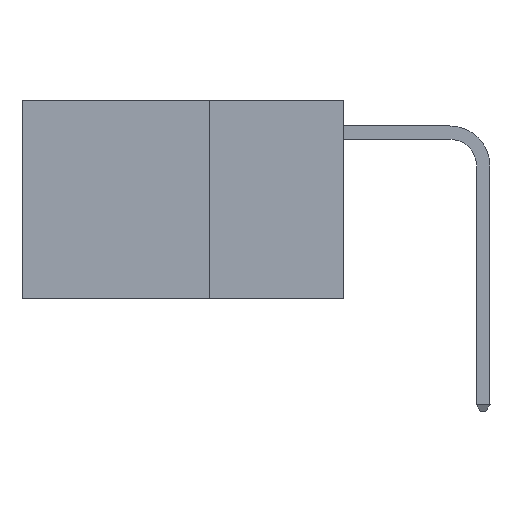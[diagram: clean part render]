
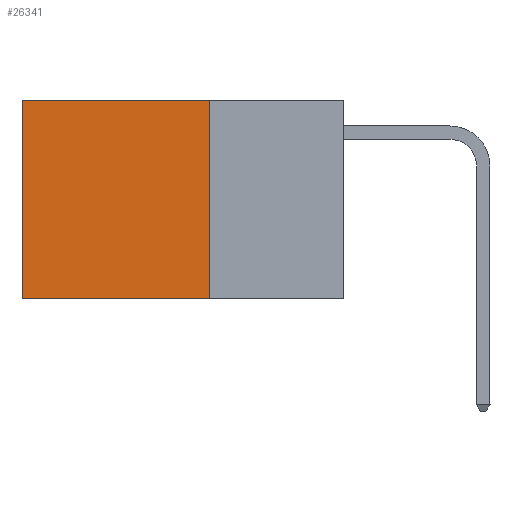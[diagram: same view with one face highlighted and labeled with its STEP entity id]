
A CAD part, left-side view. The second image highlights one B-rep face of the part: STEP entity #26341.
In plain terms, the highlighted planar face has unit normal (-1, 0, 0).
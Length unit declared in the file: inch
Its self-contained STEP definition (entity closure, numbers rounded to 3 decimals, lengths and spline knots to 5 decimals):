
#617 = ORIENTED_EDGE ( 'NONE', *, *, #25910, .F. ) ;
#640 = LINE ( 'NONE', #20412, #10256 ) ;
#1029 = LINE ( 'NONE', #9700, #5102 ) ;
#1255 = DIRECTION ( 'NONE',  ( 0., 0., -1. ) ) ;
#1884 = EDGE_CURVE ( 'NONE', #8479, #26986, #26842, .T. ) ;
#2988 = DIRECTION ( 'NONE',  ( 0., 0., -1. ) ) ;
#3360 = CARTESIAN_POINT ( 'NONE',  ( 0.2625, 0.6, 0. ) ) ;
#4978 = VERTEX_POINT ( 'NONE', #14191 ) ;
#5102 = VECTOR ( 'NONE', #18366, 39.37008 ) ;
#5733 = AXIS2_PLACEMENT_3D ( 'NONE', #16905, #27565, #8238 ) ;
#6381 = ORIENTED_EDGE ( 'NONE', *, *, #15307, .F. ) ;
#7714 = CARTESIAN_POINT ( 'NONE',  ( 0.2625, 0.25, 0. ) ) ;
#8238 = DIRECTION ( 'NONE',  ( 0., 0., -1. ) ) ;
#8479 = VERTEX_POINT ( 'NONE', #21082 ) ;
#9691 = LINE ( 'NONE', #7714, #27496 ) ;
#9700 = CARTESIAN_POINT ( 'NONE',  ( 0.2625, 0.25, 0. ) ) ;
#9746 = DIRECTION ( 'NONE',  ( 0., 1., 0. ) ) ;
#10256 = VECTOR ( 'NONE', #9746, 39.37008 ) ;
#12319 = EDGE_CURVE ( 'NONE', #15676, #8479, #1029, .T. ) ;
#13079 = ORIENTED_EDGE ( 'NONE', *, *, #1884, .T. ) ;
#14191 = CARTESIAN_POINT ( 'NONE',  ( 0.2625, 0.25, -0.37 ) ) ;
#15307 = EDGE_CURVE ( 'NONE', #15676, #4978, #9691, .T. ) ;
#15432 = EDGE_LOOP ( 'NONE', ( #13079, #617, #6381, #27812 ) ) ;
#15676 = VERTEX_POINT ( 'NONE', #27114 ) ;
#16905 = CARTESIAN_POINT ( 'NONE',  ( 0.2625, 0.25, 0. ) ) ;
#18366 = DIRECTION ( 'NONE',  ( 0., 1., 0. ) ) ;
#19162 = PLANE ( 'NONE',  #5733 ) ;
#20412 = CARTESIAN_POINT ( 'NONE',  ( 0.2625, 0.25, -0.37 ) ) ;
#21082 = CARTESIAN_POINT ( 'NONE',  ( 0.2625, 0.6, 0. ) ) ;
#23170 = VECTOR ( 'NONE', #1255, 39.37008 ) ;
#24098 = CARTESIAN_POINT ( 'NONE',  ( 0.2625, 0.6, -0.37 ) ) ;
#25910 = EDGE_CURVE ( 'NONE', #4978, #26986, #640, .T. ) ;
#26341 = ADVANCED_FACE ( 'NONE', ( #27292 ), #19162, .F. ) ;
#26842 = LINE ( 'NONE', #3360, #23170 ) ;
#26986 = VERTEX_POINT ( 'NONE', #24098 ) ;
#27114 = CARTESIAN_POINT ( 'NONE',  ( 0.2625, 0.25, 0. ) ) ;
#27292 = FACE_OUTER_BOUND ( 'NONE', #15432, .T. ) ;
#27496 = VECTOR ( 'NONE', #2988, 39.37008 ) ;
#27565 = DIRECTION ( 'NONE',  ( 1., 0., 0. ) ) ;
#27812 = ORIENTED_EDGE ( 'NONE', *, *, #12319, .T. ) ;
